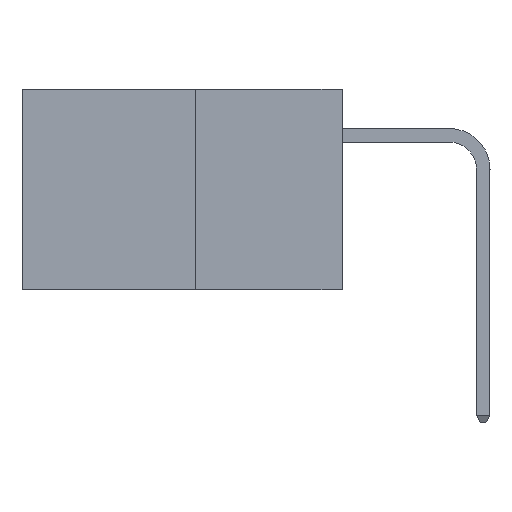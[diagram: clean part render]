
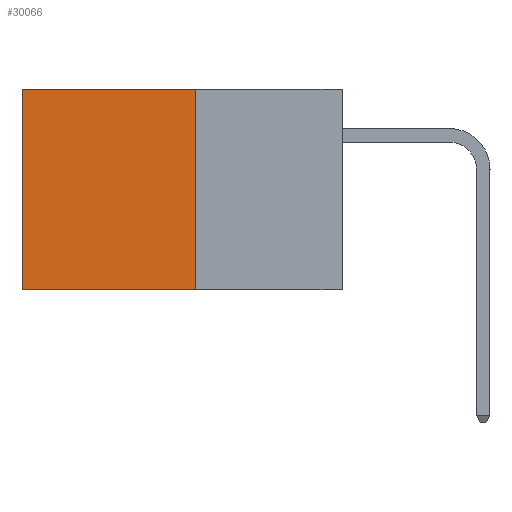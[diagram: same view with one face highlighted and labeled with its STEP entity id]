
A CAD part, left-side view. The second image highlights one B-rep face of the part: STEP entity #30066.
In plain terms, the highlighted planar face has unit normal (-1, 0, 0).
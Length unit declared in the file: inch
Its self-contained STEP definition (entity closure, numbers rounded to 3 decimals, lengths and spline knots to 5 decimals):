
#3022 = EDGE_LOOP ( 'NONE', ( #23288, #5965, #20175, #29154 ) ) ;
#3574 = CARTESIAN_POINT ( 'NONE',  ( 0.277, 0.59, -0.37 ) ) ;
#5442 = VERTEX_POINT ( 'NONE', #13683 ) ;
#5965 = ORIENTED_EDGE ( 'NONE', *, *, #10492, .F. ) ;
#6487 = VECTOR ( 'NONE', #18619, 39.37008 ) ;
#7985 = VERTEX_POINT ( 'NONE', #25911 ) ;
#8069 = LINE ( 'NONE', #16156, #6487 ) ;
#8151 = CARTESIAN_POINT ( 'NONE',  ( 0.277, 0.27, -0.37 ) ) ;
#9839 = DIRECTION ( 'NONE',  ( 0., 0., -1. ) ) ;
#10127 = CARTESIAN_POINT ( 'NONE',  ( 0.277, 0.59, -0.37 ) ) ;
#10492 = EDGE_CURVE ( 'NONE', #19577, #12248, #8069, .T. ) ;
#10522 = DIRECTION ( 'NONE',  ( 0., 1., 0. ) ) ;
#11267 = FACE_OUTER_BOUND ( 'NONE', #3022, .T. ) ;
#12248 = VERTEX_POINT ( 'NONE', #10127 ) ;
#12941 = DIRECTION ( 'NONE',  ( 0., 0., -1. ) ) ;
#13561 = EDGE_CURVE ( 'NONE', #7985, #5442, #29501, .T. ) ;
#13619 = DIRECTION ( 'NONE',  ( 0., 0., -1. ) ) ;
#13683 = CARTESIAN_POINT ( 'NONE',  ( 0.277, 0.59, 0. ) ) ;
#14126 = VECTOR ( 'NONE', #12941, 39.37008 ) ;
#15974 = LINE ( 'NONE', #3574, #28093 ) ;
#16156 = CARTESIAN_POINT ( 'NONE',  ( 0.277, 0.27, -0.37 ) ) ;
#16629 = VECTOR ( 'NONE', #10522, 39.37008 ) ;
#18619 = DIRECTION ( 'NONE',  ( 0., 1., 0. ) ) ;
#19577 = VERTEX_POINT ( 'NONE', #8151 ) ;
#19731 = PLANE ( 'NONE',  #23929 ) ;
#20175 = ORIENTED_EDGE ( 'NONE', *, *, #28329, .F. ) ;
#22122 = CARTESIAN_POINT ( 'NONE',  ( 0.277, 0.27, -0.37 ) ) ;
#23288 = ORIENTED_EDGE ( 'NONE', *, *, #23891, .T. ) ;
#23891 = EDGE_CURVE ( 'NONE', #5442, #12248, #15974, .T. ) ;
#23929 = AXIS2_PLACEMENT_3D ( 'NONE', #22122, #24555, #9839 ) ;
#24555 = DIRECTION ( 'NONE',  ( 1., 0., 0. ) ) ;
#25082 = CARTESIAN_POINT ( 'NONE',  ( 0.277, 0.27, -0.37 ) ) ;
#25911 = CARTESIAN_POINT ( 'NONE',  ( 0.277, 0.27, 0. ) ) ;
#27089 = LINE ( 'NONE', #25082, #14126 ) ;
#28093 = VECTOR ( 'NONE', #13619, 39.37008 ) ;
#28329 = EDGE_CURVE ( 'NONE', #7985, #19577, #27089, .T. ) ;
#29154 = ORIENTED_EDGE ( 'NONE', *, *, #13561, .T. ) ;
#29501 = LINE ( 'NONE', #30086, #16629 ) ;
#30066 = ADVANCED_FACE ( 'NONE', ( #11267 ), #19731, .F. ) ;
#30086 = CARTESIAN_POINT ( 'NONE',  ( 0.277, 0.27, 0. ) ) ;
